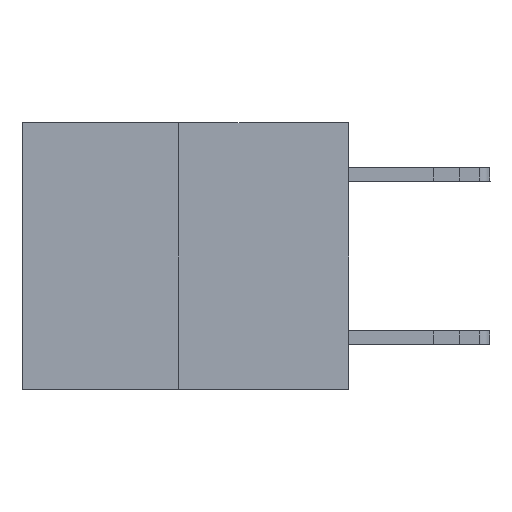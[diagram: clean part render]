
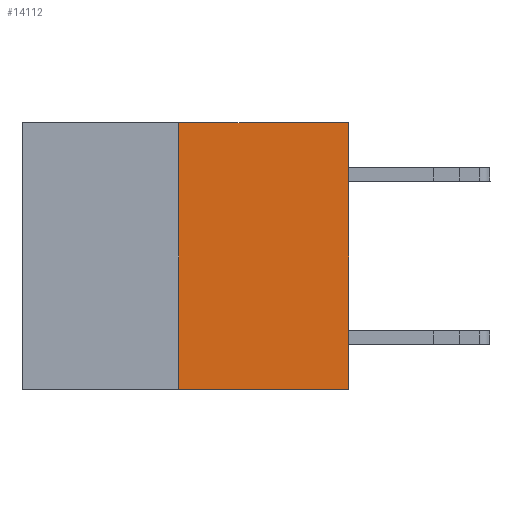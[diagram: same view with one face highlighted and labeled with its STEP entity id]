
A CAD part, left-side view. The second image highlights one B-rep face of the part: STEP entity #14112.
In plain terms, the highlighted planar face has unit normal (-1, 0, 0).
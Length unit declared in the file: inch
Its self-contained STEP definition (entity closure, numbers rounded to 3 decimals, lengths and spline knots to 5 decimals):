
#367 = EDGE_CURVE ( 'NONE', #15491, #10049, #15348, .T. ) ;
#820 = EDGE_LOOP ( 'NONE', ( #10101, #28293, #12282, #6101 ) ) ;
#2151 = FACE_OUTER_BOUND ( 'NONE', #820, .T. ) ;
#3013 = VERTEX_POINT ( 'NONE', #7911 ) ;
#3886 = VECTOR ( 'NONE', #11132, 39.37008 ) ;
#3913 = PLANE ( 'NONE',  #22053 ) ;
#5893 = LINE ( 'NONE', #20225, #17387 ) ;
#6101 = ORIENTED_EDGE ( 'NONE', *, *, #367, .F. ) ;
#6524 = DIRECTION ( 'NONE',  ( 0., -1., 0. ) ) ;
#6543 = CARTESIAN_POINT ( 'NONE',  ( 0., 0.312, -0.49 ) ) ;
#7911 = CARTESIAN_POINT ( 'NONE',  ( 0., 0.312, -0.49 ) ) ;
#9218 = CARTESIAN_POINT ( 'NONE',  ( 0., 0.6, 0. ) ) ;
#10049 = VERTEX_POINT ( 'NONE', #20638 ) ;
#10101 = ORIENTED_EDGE ( 'NONE', *, *, #21266, .F. ) ;
#11132 = DIRECTION ( 'NONE',  ( 0., 0., 1. ) ) ;
#11610 = DIRECTION ( 'NONE',  ( 0., -1., 0. ) ) ;
#12081 = VECTOR ( 'NONE', #11610, 39.37008 ) ;
#12282 = ORIENTED_EDGE ( 'NONE', *, *, #21788, .T. ) ;
#14112 = ADVANCED_FACE ( 'NONE', ( #2151 ), #3913, .F. ) ;
#15348 = LINE ( 'NONE', #9218, #12081 ) ;
#15491 = VERTEX_POINT ( 'NONE', #21228 ) ;
#16803 = VECTOR ( 'NONE', #24349, 39.37008 ) ;
#17387 = VECTOR ( 'NONE', #6524, 39.37008 ) ;
#17429 = CARTESIAN_POINT ( 'NONE',  ( 0., 0., 0. ) ) ;
#17564 = LINE ( 'NONE', #6543, #3886 ) ;
#17896 = EDGE_CURVE ( 'NONE', #3013, #20352, #5893, .T. ) ;
#19221 = CARTESIAN_POINT ( 'NONE',  ( 0., 0., -0.49 ) ) ;
#20125 = DIRECTION ( 'NONE',  ( 0., 0., -1. ) ) ;
#20225 = CARTESIAN_POINT ( 'NONE',  ( 0., 0.6, -0.49 ) ) ;
#20352 = VERTEX_POINT ( 'NONE', #19221 ) ;
#20638 = CARTESIAN_POINT ( 'NONE',  ( 0., 0., 0. ) ) ;
#21228 = CARTESIAN_POINT ( 'NONE',  ( 0., 0.312, 0. ) ) ;
#21266 = EDGE_CURVE ( 'NONE', #3013, #15491, #17564, .T. ) ;
#21788 = EDGE_CURVE ( 'NONE', #20352, #10049, #28980, .T. ) ;
#22053 = AXIS2_PLACEMENT_3D ( 'NONE', #28696, #22215, #20125 ) ;
#22215 = DIRECTION ( 'NONE',  ( 1., 0., 0. ) ) ;
#24349 = DIRECTION ( 'NONE',  ( 0., 0., 1. ) ) ;
#28293 = ORIENTED_EDGE ( 'NONE', *, *, #17896, .T. ) ;
#28696 = CARTESIAN_POINT ( 'NONE',  ( 0., 0.6, 0. ) ) ;
#28980 = LINE ( 'NONE', #17429, #16803 ) ;
